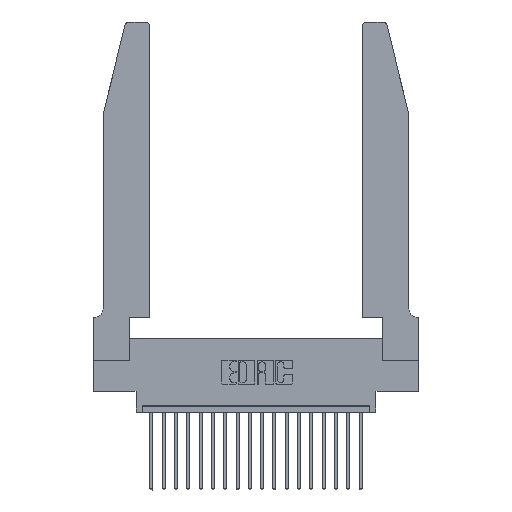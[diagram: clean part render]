
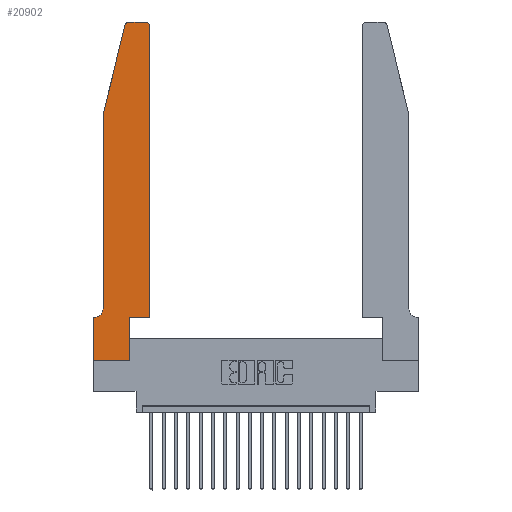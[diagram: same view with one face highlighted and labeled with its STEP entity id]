
A CAD part, top view. The second image highlights one B-rep face of the part: STEP entity #20902.
In plain terms, the highlighted planar face has unit normal (0, 0, 1).
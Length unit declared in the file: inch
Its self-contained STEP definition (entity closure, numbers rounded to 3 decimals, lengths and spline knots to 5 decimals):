
#210 = LINE ( 'NONE', #1568, #13063 ) ;
#344 = CARTESIAN_POINT ( 'NONE',  ( 0.0755, 0.35, 0.37 ) ) ;
#359 = VECTOR ( 'NONE', #16094, 39.37008 ) ;
#901 = AXIS2_PLACEMENT_3D ( 'NONE', #16956, #5405, #10540 ) ;
#1142 = CIRCLE ( 'NONE', #17122, 0.07 ) ;
#1568 = CARTESIAN_POINT ( 'NONE',  ( 0., 0., 0.37 ) ) ;
#1661 = CARTESIAN_POINT ( 'NONE',  ( 0.0055, 0.35, 0.37 ) ) ;
#1940 = EDGE_CURVE ( 'NONE', #3061, #12069, #7990, .T. ) ;
#2387 = CARTESIAN_POINT ( 'NONE',  ( 0.0755, 2., 0.37 ) ) ;
#2822 = VECTOR ( 'NONE', #9638, 39.37008 ) ;
#3061 = VERTEX_POINT ( 'NONE', #20784 ) ;
#3335 = CARTESIAN_POINT ( 'NONE',  ( 0.4205, 2.72, 0.37 ) ) ;
#3554 = VECTOR ( 'NONE', #7004, 39.37008 ) ;
#4007 = ORIENTED_EDGE ( 'NONE', *, *, #13527, .T. ) ;
#4058 = CARTESIAN_POINT ( 'NONE',  ( 0.25487, 2.72718, 0.37 ) ) ;
#4149 = ORIENTED_EDGE ( 'NONE', *, *, #18120, .T. ) ;
#4821 = FACE_OUTER_BOUND ( 'NONE', #19036, .T. ) ;
#4841 = LINE ( 'NONE', #9307, #359 ) ;
#5062 = CARTESIAN_POINT ( 'NONE',  ( 0.0755, 0.42, 0.37 ) ) ;
#5283 = CIRCLE ( 'NONE', #9440, 0.03 ) ;
#5405 = DIRECTION ( 'NONE',  ( 0., 0., 1. ) ) ;
#5509 = DIRECTION ( 'NONE',  ( 0., 1., 0. ) ) ;
#5765 = ORIENTED_EDGE ( 'NONE', *, *, #6318, .T. ) ;
#5862 = EDGE_CURVE ( 'NONE', #10569, #3061, #210, .T. ) ;
#6126 = CARTESIAN_POINT ( 'NONE',  ( 0.284, 2.72, 0.37 ) ) ;
#6184 = VERTEX_POINT ( 'NONE', #14592 ) ;
#6306 = EDGE_CURVE ( 'NONE', #10392, #10569, #6529, .T. ) ;
#6318 = EDGE_CURVE ( 'NONE', #9507, #19719, #20328, .T. ) ;
#6327 = CARTESIAN_POINT ( 'NONE',  ( 0.2865, 0.35, 0.37 ) ) ;
#6480 = DIRECTION ( 'NONE',  ( -1., 0., 0. ) ) ;
#6529 = LINE ( 'NONE', #13919, #15917 ) ;
#7004 = DIRECTION ( 'NONE',  ( -1., 0., 0. ) ) ;
#7148 = CARTESIAN_POINT ( 'NONE',  ( 0.4505, 0.35, 0.37 ) ) ;
#7243 = EDGE_CURVE ( 'NONE', #13020, #10392, #10383, .T. ) ;
#7321 = VERTEX_POINT ( 'NONE', #8292 ) ;
#7990 = LINE ( 'NONE', #6327, #16350 ) ;
#8074 = EDGE_CURVE ( 'NONE', #20652, #13020, #1142, .T. ) ;
#8235 = CARTESIAN_POINT ( 'NONE',  ( 0.4505, 0.35, 0.37 ) ) ;
#8292 = CARTESIAN_POINT ( 'NONE',  ( 0.284, 2.75, 0.37 ) ) ;
#8399 = ORIENTED_EDGE ( 'NONE', *, *, #12120, .T. ) ;
#9279 = VERTEX_POINT ( 'NONE', #21404 ) ;
#9307 = CARTESIAN_POINT ( 'NONE',  ( 0.0755, 2., 0.37 ) ) ;
#9440 = AXIS2_PLACEMENT_3D ( 'NONE', #3335, #13441, #10209 ) ;
#9481 = DIRECTION ( 'NONE',  ( 1., 0., 0. ) ) ;
#9507 = VERTEX_POINT ( 'NONE', #11950 ) ;
#9638 = DIRECTION ( 'NONE',  ( 1., 0., 0. ) ) ;
#9660 = LINE ( 'NONE', #8235, #2822 ) ;
#9668 = CARTESIAN_POINT ( 'NONE',  ( 0., 0., 0.37 ) ) ;
#9705 = ORIENTED_EDGE ( 'NONE', *, *, #1940, .T. ) ;
#9877 = ORIENTED_EDGE ( 'NONE', *, *, #5862, .T. ) ;
#10209 = DIRECTION ( 'NONE',  ( 1., 0., 0. ) ) ;
#10383 = LINE ( 'NONE', #344, #15350 ) ;
#10392 = VERTEX_POINT ( 'NONE', #12099 ) ;
#10504 = CARTESIAN_POINT ( 'NONE',  ( 0.4505, 2.72, 0.37 ) ) ;
#10540 = DIRECTION ( 'NONE',  ( 1., 0., 0. ) ) ;
#10569 = VERTEX_POINT ( 'NONE', #9668 ) ;
#10619 = LINE ( 'NONE', #2387, #18960 ) ;
#10697 = ORIENTED_EDGE ( 'NONE', *, *, #11127, .T. ) ;
#10732 = CIRCLE ( 'NONE', #18269, 0.03 ) ;
#11127 = EDGE_CURVE ( 'NONE', #7321, #11651, #10732, .T. ) ;
#11641 = DIRECTION ( 'NONE',  ( 0., 0., -1. ) ) ;
#11651 = VERTEX_POINT ( 'NONE', #4058 ) ;
#11950 = CARTESIAN_POINT ( 'NONE',  ( 0.4505, 0.35, 0.37 ) ) ;
#12069 = VERTEX_POINT ( 'NONE', #16255 ) ;
#12099 = CARTESIAN_POINT ( 'NONE',  ( 0., 0.35, 0.37 ) ) ;
#12120 = EDGE_CURVE ( 'NONE', #12069, #9507, #9660, .T. ) ;
#12165 = CARTESIAN_POINT ( 'NONE',  ( 0.2605, 2.75, 0.37 ) ) ;
#13020 = VERTEX_POINT ( 'NONE', #1661 ) ;
#13047 = ORIENTED_EDGE ( 'NONE', *, *, #6306, .T. ) ;
#13063 = VECTOR ( 'NONE', #16549, 39.37008 ) ;
#13105 = EDGE_CURVE ( 'NONE', #9279, #7321, #14820, .T. ) ;
#13441 = DIRECTION ( 'NONE',  ( 0., 0., 1. ) ) ;
#13527 = EDGE_CURVE ( 'NONE', #11651, #6184, #10619, .T. ) ;
#13651 = EDGE_CURVE ( 'NONE', #6184, #20652, #4841, .T. ) ;
#13669 = ORIENTED_EDGE ( 'NONE', *, *, #13105, .T. ) ;
#13754 = PLANE ( 'NONE',  #901 ) ;
#13818 = VECTOR ( 'NONE', #5509, 39.37008 ) ;
#13897 = DIRECTION ( 'NONE',  ( -1., 0., 0. ) ) ;
#13919 = CARTESIAN_POINT ( 'NONE',  ( 0., 0., 0.37 ) ) ;
#14592 = CARTESIAN_POINT ( 'NONE',  ( 0.0755, 2., 0.37 ) ) ;
#14697 = DIRECTION ( 'NONE',  ( 0., 1., 0. ) ) ;
#14820 = LINE ( 'NONE', #12165, #3554 ) ;
#15325 = ORIENTED_EDGE ( 'NONE', *, *, #13651, .T. ) ;
#15350 = VECTOR ( 'NONE', #13897, 39.37008 ) ;
#15917 = VECTOR ( 'NONE', #20698, 39.37008 ) ;
#16094 = DIRECTION ( 'NONE',  ( 0., -1., 0. ) ) ;
#16172 = DIRECTION ( 'NONE',  ( -0.239, -0.971, 0. ) ) ;
#16187 = ORIENTED_EDGE ( 'NONE', *, *, #7243, .T. ) ;
#16255 = CARTESIAN_POINT ( 'NONE',  ( 0.2865, 0.35, 0.37 ) ) ;
#16350 = VECTOR ( 'NONE', #14697, 39.37008 ) ;
#16549 = DIRECTION ( 'NONE',  ( 1., 0., 0. ) ) ;
#16956 = CARTESIAN_POINT ( 'NONE',  ( 0., 0.35, 0.37 ) ) ;
#17122 = AXIS2_PLACEMENT_3D ( 'NONE', #18057, #11641, #6480 ) ;
#17303 = ORIENTED_EDGE ( 'NONE', *, *, #8074, .T. ) ;
#17784 = DIRECTION ( 'NONE',  ( 0., 0., 1. ) ) ;
#18057 = CARTESIAN_POINT ( 'NONE',  ( 0.0055, 0.42, 0.37 ) ) ;
#18120 = EDGE_CURVE ( 'NONE', #19719, #9279, #5283, .T. ) ;
#18269 = AXIS2_PLACEMENT_3D ( 'NONE', #6126, #17784, #9481 ) ;
#18960 = VECTOR ( 'NONE', #16172, 39.37008 ) ;
#19036 = EDGE_LOOP ( 'NONE', ( #13669, #10697, #4007, #15325, #17303, #16187, #13047, #9877, #9705, #8399, #5765, #4149 ) ) ;
#19719 = VERTEX_POINT ( 'NONE', #10504 ) ;
#20328 = LINE ( 'NONE', #7148, #13818 ) ;
#20652 = VERTEX_POINT ( 'NONE', #5062 ) ;
#20698 = DIRECTION ( 'NONE',  ( 0., -1., 0. ) ) ;
#20784 = CARTESIAN_POINT ( 'NONE',  ( 0.2865, 0., 0.37 ) ) ;
#20902 = ADVANCED_FACE ( 'NONE', ( #4821 ), #13754, .T. ) ;
#21404 = CARTESIAN_POINT ( 'NONE',  ( 0.4205, 2.75, 0.37 ) ) ;
